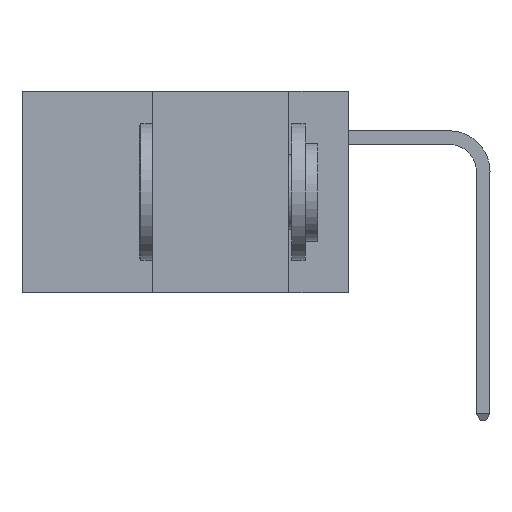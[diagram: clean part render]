
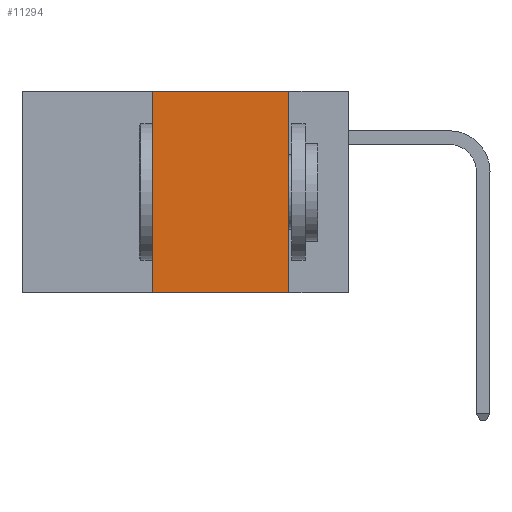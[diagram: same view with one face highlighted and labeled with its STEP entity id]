
A CAD part, left-side view. The second image highlights one B-rep face of the part: STEP entity #11294.
In plain terms, the highlighted planar face has unit normal (-1, 0, 0).
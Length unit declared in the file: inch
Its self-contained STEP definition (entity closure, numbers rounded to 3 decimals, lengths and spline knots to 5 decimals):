
#977 = VERTEX_POINT ( 'NONE', #10135 ) ;
#995 = DIRECTION ( 'NONE',  ( 0., -1., 0. ) ) ;
#3001 = EDGE_LOOP ( 'NONE', ( #6678, #8034, #8880, #9560 ) ) ;
#3316 = CARTESIAN_POINT ( 'NONE',  ( 0., 0.6, 0. ) ) ;
#3432 = LINE ( 'NONE', #21694, #21123 ) ;
#4764 = FACE_OUTER_BOUND ( 'NONE', #3001, .T. ) ;
#5281 = DIRECTION ( 'NONE',  ( 1., 0., 0. ) ) ;
#5997 = LINE ( 'NONE', #24388, #21508 ) ;
#6489 = LINE ( 'NONE', #8067, #11614 ) ;
#6535 = CARTESIAN_POINT ( 'NONE',  ( 0., 0.11, 0. ) ) ;
#6678 = ORIENTED_EDGE ( 'NONE', *, *, #21236, .F. ) ;
#8034 = ORIENTED_EDGE ( 'NONE', *, *, #24400, .F. ) ;
#8067 = CARTESIAN_POINT ( 'NONE',  ( 0., 0.6, -0.37 ) ) ;
#8757 = CARTESIAN_POINT ( 'NONE',  ( 0., 0.11, -0.37 ) ) ;
#8880 = ORIENTED_EDGE ( 'NONE', *, *, #10786, .F. ) ;
#9560 = ORIENTED_EDGE ( 'NONE', *, *, #15086, .T. ) ;
#10135 = CARTESIAN_POINT ( 'NONE',  ( 0., 0.36, 0. ) ) ;
#10692 = AXIS2_PLACEMENT_3D ( 'NONE', #3316, #5281, #18500 ) ;
#10786 = EDGE_CURVE ( 'NONE', #15610, #977, #5997, .T. ) ;
#11294 = ADVANCED_FACE ( 'NONE', ( #4764 ), #14786, .F. ) ;
#11504 = DIRECTION ( 'NONE',  ( 0., 0., 1. ) ) ;
#11614 = VECTOR ( 'NONE', #19205, 39.37008 ) ;
#11827 = CARTESIAN_POINT ( 'NONE',  ( 0., 0.11, 0. ) ) ;
#14786 = PLANE ( 'NONE',  #10692 ) ;
#15086 = EDGE_CURVE ( 'NONE', #15610, #16344, #6489, .T. ) ;
#15610 = VERTEX_POINT ( 'NONE', #18943 ) ;
#16344 = VERTEX_POINT ( 'NONE', #8757 ) ;
#18041 = VERTEX_POINT ( 'NONE', #6535 ) ;
#18500 = DIRECTION ( 'NONE',  ( 0., 0., -1. ) ) ;
#18943 = CARTESIAN_POINT ( 'NONE',  ( 0., 0.36, -0.37 ) ) ;
#19205 = DIRECTION ( 'NONE',  ( 0., -1., 0. ) ) ;
#19238 = DIRECTION ( 'NONE',  ( 0., 0., -1. ) ) ;
#20409 = VECTOR ( 'NONE', #19238, 39.37008 ) ;
#21000 = LINE ( 'NONE', #11827, #20409 ) ;
#21123 = VECTOR ( 'NONE', #995, 39.37008 ) ;
#21236 = EDGE_CURVE ( 'NONE', #18041, #16344, #21000, .T. ) ;
#21508 = VECTOR ( 'NONE', #11504, 39.37008 ) ;
#21694 = CARTESIAN_POINT ( 'NONE',  ( 0., 0.6, 0. ) ) ;
#24388 = CARTESIAN_POINT ( 'NONE',  ( 0., 0.36, 0. ) ) ;
#24400 = EDGE_CURVE ( 'NONE', #977, #18041, #3432, .T. ) ;
